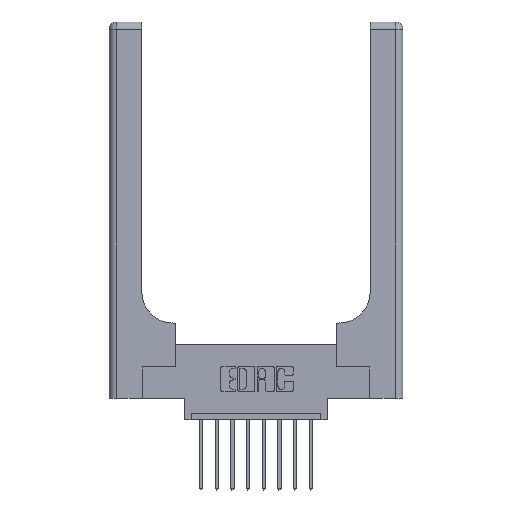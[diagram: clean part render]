
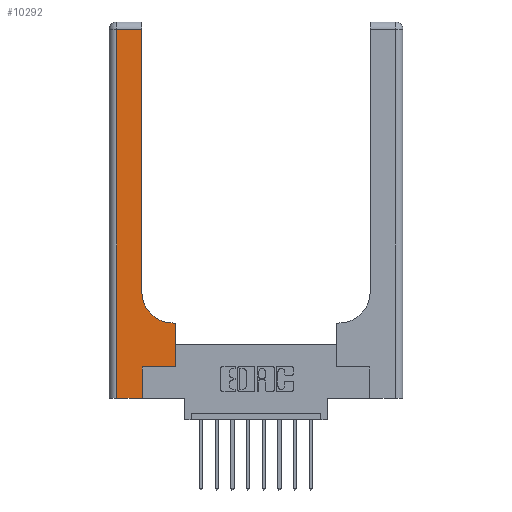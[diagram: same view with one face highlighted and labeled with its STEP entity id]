
A CAD part, top view. The second image highlights one B-rep face of the part: STEP entity #10292.
In plain terms, the highlighted planar face has unit normal (0, 0, 1).
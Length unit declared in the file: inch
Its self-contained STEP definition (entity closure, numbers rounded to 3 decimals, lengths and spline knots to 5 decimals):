
#122 = CARTESIAN_POINT ( 'NONE',  ( 0.265, 0., 0.37 ) ) ;
#531 = EDGE_LOOP ( 'NONE', ( #12741, #11550, #12869, #1213, #6806, #8410, #13907, #13669, #9635 ) ) ;
#559 = CARTESIAN_POINT ( 'NONE',  ( 0., 2.94, 0.37 ) ) ;
#626 = CARTESIAN_POINT ( 'NONE',  ( 0.51, 0.85, 0.37 ) ) ;
#721 = CARTESIAN_POINT ( 'NONE',  ( 0.265, 0.25, 0.37 ) ) ;
#859 = DIRECTION ( 'NONE',  ( 1., 0., 0. ) ) ;
#1111 = CARTESIAN_POINT ( 'NONE',  ( 0.26, 3., 0.37 ) ) ;
#1213 = ORIENTED_EDGE ( 'NONE', *, *, #1659, .T. ) ;
#1659 = EDGE_CURVE ( 'NONE', #7209, #6069, #2005, .T. ) ;
#2005 = LINE ( 'NONE', #10266, #5384 ) ;
#2007 = CARTESIAN_POINT ( 'NONE',  ( 0., 3., 0.37 ) ) ;
#2296 = VERTEX_POINT ( 'NONE', #2721 ) ;
#2721 = CARTESIAN_POINT ( 'NONE',  ( 0.26, 2.94, 0.37 ) ) ;
#2986 = VECTOR ( 'NONE', #9752, 39.37008 ) ;
#3021 = PLANE ( 'NONE',  #15215 ) ;
#3137 = EDGE_CURVE ( 'NONE', #7990, #14893, #3737, .T. ) ;
#3143 = CIRCLE ( 'NONE', #11756, 0.25 ) ;
#3162 = DIRECTION ( 'NONE',  ( -1., 0., 0. ) ) ;
#3312 = FACE_OUTER_BOUND ( 'NONE', #531, .T. ) ;
#3314 = CARTESIAN_POINT ( 'NONE',  ( 0.265, 0.25, 0.37 ) ) ;
#3410 = CARTESIAN_POINT ( 'NONE',  ( 0.528, 0.25, 0.37 ) ) ;
#3607 = CARTESIAN_POINT ( 'NONE',  ( 0.06, 2.94, 0.37 ) ) ;
#3734 = EDGE_CURVE ( 'NONE', #14893, #12607, #7976, .T. ) ;
#3737 = LINE ( 'NONE', #8433, #6811 ) ;
#4431 = EDGE_CURVE ( 'NONE', #4816, #7209, #12439, .T. ) ;
#4433 = LINE ( 'NONE', #9130, #14630 ) ;
#4816 = VERTEX_POINT ( 'NONE', #3607 ) ;
#5031 = LINE ( 'NONE', #559, #2986 ) ;
#5384 = VECTOR ( 'NONE', #15000, 39.37008 ) ;
#5433 = CARTESIAN_POINT ( 'NONE',  ( 0.51, 0.6, 0.37 ) ) ;
#6069 = VERTEX_POINT ( 'NONE', #122 ) ;
#6806 = ORIENTED_EDGE ( 'NONE', *, *, #13918, .T. ) ;
#6811 = VECTOR ( 'NONE', #9689, 39.37008 ) ;
#6819 = VECTOR ( 'NONE', #8217, 39.37008 ) ;
#6910 = DIRECTION ( 'NONE',  ( -1., 0., 0. ) ) ;
#7209 = VERTEX_POINT ( 'NONE', #12065 ) ;
#7338 = DIRECTION ( 'NONE',  ( 1., 0., 0. ) ) ;
#7786 = DIRECTION ( 'NONE',  ( 0., 0., -1. ) ) ;
#7801 = LINE ( 'NONE', #721, #14295 ) ;
#7976 = LINE ( 'NONE', #12762, #9554 ) ;
#7990 = VERTEX_POINT ( 'NONE', #3410 ) ;
#8217 = DIRECTION ( 'NONE',  ( 0., 1., 0. ) ) ;
#8410 = ORIENTED_EDGE ( 'NONE', *, *, #8965, .T. ) ;
#8433 = CARTESIAN_POINT ( 'NONE',  ( 0.528, 0.25, 0.37 ) ) ;
#8965 = EDGE_CURVE ( 'NONE', #11457, #7990, #7801, .T. ) ;
#9130 = CARTESIAN_POINT ( 'NONE',  ( 0.265, 0., 0.37 ) ) ;
#9554 = VECTOR ( 'NONE', #6910, 39.37008 ) ;
#9635 = ORIENTED_EDGE ( 'NONE', *, *, #10247, .T. ) ;
#9684 = EDGE_CURVE ( 'NONE', #14172, #2296, #10837, .T. ) ;
#9689 = DIRECTION ( 'NONE',  ( 0., 1., 0. ) ) ;
#9752 = DIRECTION ( 'NONE',  ( -1., 0., 0. ) ) ;
#10001 = CARTESIAN_POINT ( 'NONE',  ( 0.06, 3., 0.37 ) ) ;
#10247 = EDGE_CURVE ( 'NONE', #12607, #14172, #3143, .T. ) ;
#10266 = CARTESIAN_POINT ( 'NONE',  ( 0., 0., 0.37 ) ) ;
#10292 = ADVANCED_FACE ( 'NONE', ( #3312 ), #3021, .F. ) ;
#10472 = CARTESIAN_POINT ( 'NONE',  ( 0.528, 0.6, 0.37 ) ) ;
#10755 = CARTESIAN_POINT ( 'NONE',  ( 0.26, 0.85, 0.37 ) ) ;
#10837 = LINE ( 'NONE', #1111, #6819 ) ;
#11048 = DIRECTION ( 'NONE',  ( 0., 0., -1. ) ) ;
#11213 = EDGE_CURVE ( 'NONE', #2296, #4816, #5031, .T. ) ;
#11457 = VERTEX_POINT ( 'NONE', #3314 ) ;
#11550 = ORIENTED_EDGE ( 'NONE', *, *, #11213, .T. ) ;
#11756 = AXIS2_PLACEMENT_3D ( 'NONE', #626, #11048, #7338 ) ;
#12065 = CARTESIAN_POINT ( 'NONE',  ( 0.06, 0., 0.37 ) ) ;
#12439 = LINE ( 'NONE', #10001, #15102 ) ;
#12607 = VERTEX_POINT ( 'NONE', #5433 ) ;
#12741 = ORIENTED_EDGE ( 'NONE', *, *, #9684, .T. ) ;
#12762 = CARTESIAN_POINT ( 'NONE',  ( 0.26, 0.6, 0.37 ) ) ;
#12869 = ORIENTED_EDGE ( 'NONE', *, *, #4431, .T. ) ;
#13669 = ORIENTED_EDGE ( 'NONE', *, *, #3734, .T. ) ;
#13907 = ORIENTED_EDGE ( 'NONE', *, *, #3137, .T. ) ;
#13916 = DIRECTION ( 'NONE',  ( 0., 1., 0. ) ) ;
#13918 = EDGE_CURVE ( 'NONE', #6069, #11457, #4433, .T. ) ;
#14172 = VERTEX_POINT ( 'NONE', #10755 ) ;
#14295 = VECTOR ( 'NONE', #859, 39.37008 ) ;
#14630 = VECTOR ( 'NONE', #13916, 39.37008 ) ;
#14873 = DIRECTION ( 'NONE',  ( 0., -1., 0. ) ) ;
#14893 = VERTEX_POINT ( 'NONE', #10472 ) ;
#15000 = DIRECTION ( 'NONE',  ( 1., 0., 0. ) ) ;
#15102 = VECTOR ( 'NONE', #14873, 39.37008 ) ;
#15215 = AXIS2_PLACEMENT_3D ( 'NONE', #2007, #7786, #3162 ) ;
